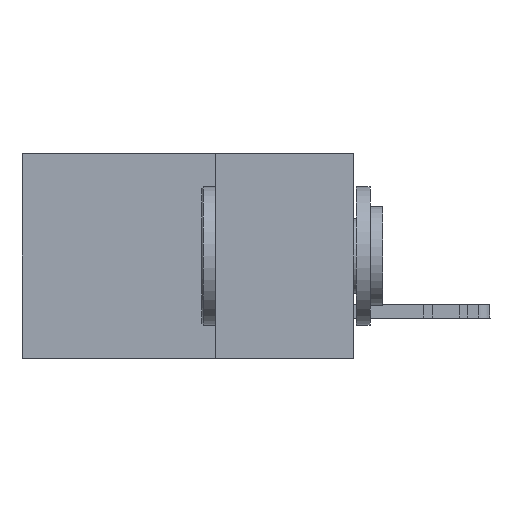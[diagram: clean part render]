
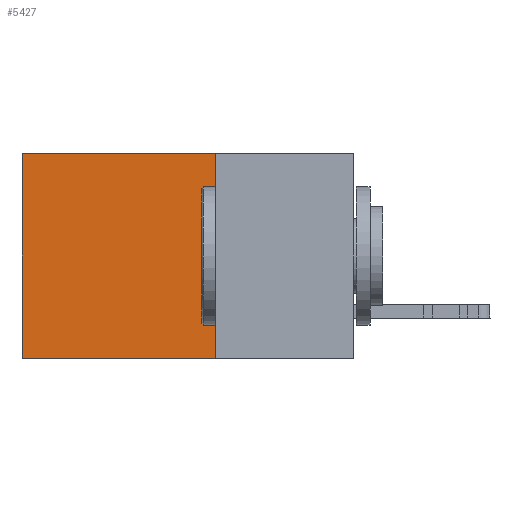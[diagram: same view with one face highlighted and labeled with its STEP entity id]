
A CAD part, left-side view. The second image highlights one B-rep face of the part: STEP entity #5427.
In plain terms, the highlighted planar face has unit normal (-1, 0, 0).
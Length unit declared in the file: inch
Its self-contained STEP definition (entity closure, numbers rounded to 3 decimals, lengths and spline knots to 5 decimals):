
#930 = VECTOR ( 'NONE', #26181, 39.37008 ) ;
#1869 = CARTESIAN_POINT ( 'NONE',  ( 0.2875, 0.25, 0. ) ) ;
#2492 = CARTESIAN_POINT ( 'NONE',  ( 0.2875, 0.25, -0.37 ) ) ;
#4082 = DIRECTION ( 'NONE',  ( 0., 0., -1. ) ) ;
#5427 = ADVANCED_FACE ( 'NONE', ( #15273 ), #23984, .F. ) ;
#6843 = CARTESIAN_POINT ( 'NONE',  ( 0.2875, 0.25, -0.37 ) ) ;
#7332 = EDGE_LOOP ( 'NONE', ( #30437, #31461, #22854, #29118 ) ) ;
#7779 = CARTESIAN_POINT ( 'NONE',  ( 0.2875, 0.25, 0. ) ) ;
#9243 = VECTOR ( 'NONE', #41344, 39.37008 ) ;
#10293 = CARTESIAN_POINT ( 'NONE',  ( 0.2875, 0.25, 0. ) ) ;
#10418 = VECTOR ( 'NONE', #4082, 39.37008 ) ;
#10823 = LINE ( 'NONE', #7779, #930 ) ;
#14405 = VERTEX_POINT ( 'NONE', #2492 ) ;
#14575 = EDGE_CURVE ( 'NONE', #14405, #17001, #43652, .T. ) ;
#15026 = CARTESIAN_POINT ( 'NONE',  ( 0.2875, 0.6, 0. ) ) ;
#15273 = FACE_OUTER_BOUND ( 'NONE', #7332, .T. ) ;
#17001 = VERTEX_POINT ( 'NONE', #26538 ) ;
#18610 = CARTESIAN_POINT ( 'NONE',  ( 0.2875, 0.6, 0. ) ) ;
#20684 = VECTOR ( 'NONE', #48172, 39.37008 ) ;
#21782 = VERTEX_POINT ( 'NONE', #18610 ) ;
#22854 = ORIENTED_EDGE ( 'NONE', *, *, #40620, .F. ) ;
#23984 = PLANE ( 'NONE',  #41038 ) ;
#24949 = DIRECTION ( 'NONE',  ( 0., 0., -1. ) ) ;
#26181 = DIRECTION ( 'NONE',  ( 0., 1., 0. ) ) ;
#26538 = CARTESIAN_POINT ( 'NONE',  ( 0.2875, 0.6, -0.37 ) ) ;
#28058 = DIRECTION ( 'NONE',  ( 1., 0., 0. ) ) ;
#29118 = ORIENTED_EDGE ( 'NONE', *, *, #40140, .T. ) ;
#30437 = ORIENTED_EDGE ( 'NONE', *, *, #36602, .T. ) ;
#31461 = ORIENTED_EDGE ( 'NONE', *, *, #14575, .F. ) ;
#32881 = LINE ( 'NONE', #33621, #20684 ) ;
#33621 = CARTESIAN_POINT ( 'NONE',  ( 0.2875, 0.25, 0. ) ) ;
#36602 = EDGE_CURVE ( 'NONE', #21782, #17001, #37752, .T. ) ;
#37752 = LINE ( 'NONE', #15026, #10418 ) ;
#40140 = EDGE_CURVE ( 'NONE', #43357, #21782, #10823, .T. ) ;
#40620 = EDGE_CURVE ( 'NONE', #43357, #14405, #32881, .T. ) ;
#41038 = AXIS2_PLACEMENT_3D ( 'NONE', #1869, #28058, #24949 ) ;
#41344 = DIRECTION ( 'NONE',  ( 0., 1., 0. ) ) ;
#43357 = VERTEX_POINT ( 'NONE', #10293 ) ;
#43652 = LINE ( 'NONE', #6843, #9243 ) ;
#48172 = DIRECTION ( 'NONE',  ( 0., 0., -1. ) ) ;
